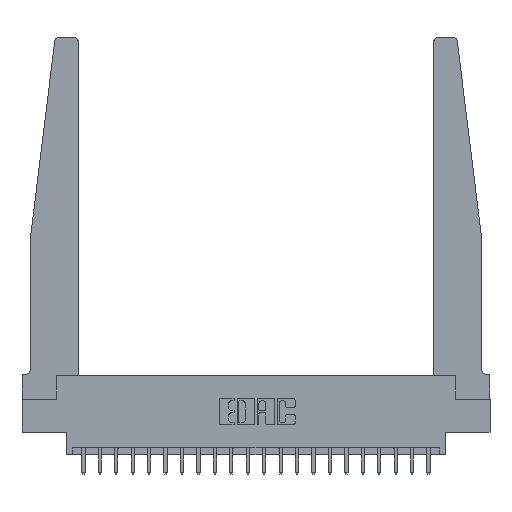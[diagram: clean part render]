
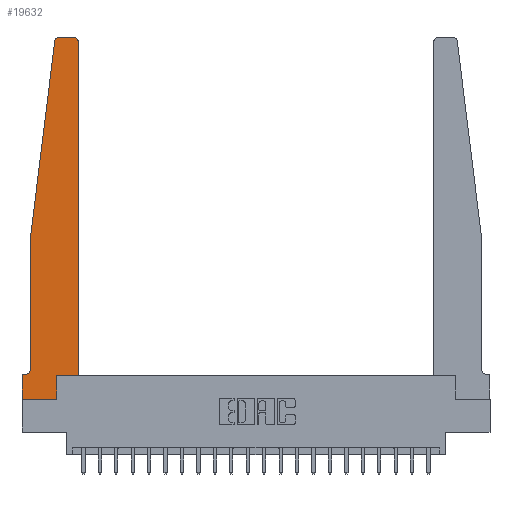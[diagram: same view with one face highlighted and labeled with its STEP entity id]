
A CAD part, top view. The second image highlights one B-rep face of the part: STEP entity #19632.
In plain terms, the highlighted planar face has unit normal (0, 0, 1).
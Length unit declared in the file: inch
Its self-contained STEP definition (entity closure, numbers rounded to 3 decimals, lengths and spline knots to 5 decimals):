
#155 = EDGE_CURVE ( 'NONE', #15139, #5308, #11760, .T. ) ;
#299 = ORIENTED_EDGE ( 'NONE', *, *, #3177, .T. ) ;
#347 = ORIENTED_EDGE ( 'NONE', *, *, #19685, .T. ) ;
#627 = VERTEX_POINT ( 'NONE', #21850 ) ;
#739 = ORIENTED_EDGE ( 'NONE', *, *, #18659, .T. ) ;
#1075 = DIRECTION ( 'NONE',  ( -1., 0., 0. ) ) ;
#1211 = CARTESIAN_POINT ( 'NONE',  ( 0.25, 2.75, 0.37 ) ) ;
#1256 = DIRECTION ( 'NONE',  ( 1., 0., 0. ) ) ;
#1295 = VECTOR ( 'NONE', #15634, 39.37008 ) ;
#1344 = DIRECTION ( 'NONE',  ( -0.122, -0.992, 0. ) ) ;
#1423 = VECTOR ( 'NONE', #5799, 39.37008 ) ;
#1841 = EDGE_CURVE ( 'NONE', #19586, #11223, #8294, .T. ) ;
#2174 = CARTESIAN_POINT ( 'NONE',  ( 0.27653, 2.75, 0.37 ) ) ;
#2571 = VECTOR ( 'NONE', #12663, 39.37008 ) ;
#2574 = LINE ( 'NONE', #14604, #6746 ) ;
#2697 = CARTESIAN_POINT ( 'NONE',  ( 0., 0., 0.37 ) ) ;
#2795 = ORIENTED_EDGE ( 'NONE', *, *, #12098, .T. ) ;
#2828 = EDGE_CURVE ( 'NONE', #16795, #3503, #19050, .T. ) ;
#3177 = EDGE_CURVE ( 'NONE', #13817, #21384, #4140, .T. ) ;
#3387 = ORIENTED_EDGE ( 'NONE', *, *, #6261, .T. ) ;
#3472 = CARTESIAN_POINT ( 'NONE',  ( 0.24675, 2.72367, 0.37 ) ) ;
#3503 = VERTEX_POINT ( 'NONE', #15905 ) ;
#3521 = ORIENTED_EDGE ( 'NONE', *, *, #12812, .T. ) ;
#3889 = DIRECTION ( 'NONE',  ( 1., 0., 0. ) ) ;
#4140 = LINE ( 'NONE', #8401, #17217 ) ;
#4718 = EDGE_LOOP ( 'NONE', ( #5007, #3387, #2795, #13019, #3521, #19135, #5939, #299, #347, #12389, #6267, #739 ) ) ;
#4885 = CARTESIAN_POINT ( 'NONE',  ( 0.065, 0.1875, 0.37 ) ) ;
#5007 = ORIENTED_EDGE ( 'NONE', *, *, #155, .T. ) ;
#5148 = VERTEX_POINT ( 'NONE', #3472 ) ;
#5308 = VERTEX_POINT ( 'NONE', #2174 ) ;
#5482 = CARTESIAN_POINT ( 'NONE',  ( 0., 0., 0.37 ) ) ;
#5781 = LINE ( 'NONE', #16782, #18746 ) ;
#5799 = DIRECTION ( 'NONE',  ( 0., -1., 0. ) ) ;
#5852 = CARTESIAN_POINT ( 'NONE',  ( 0.065, 1.25, 0.37 ) ) ;
#5927 = EDGE_CURVE ( 'NONE', #627, #13817, #10507, .T. ) ;
#5939 = ORIENTED_EDGE ( 'NONE', *, *, #5927, .T. ) ;
#5998 = CARTESIAN_POINT ( 'NONE',  ( 0.425, 0.18, 0.37 ) ) ;
#6261 = EDGE_CURVE ( 'NONE', #5308, #5148, #9170, .T. ) ;
#6266 = CIRCLE ( 'NONE', #16743, 0.03 ) ;
#6267 = ORIENTED_EDGE ( 'NONE', *, *, #8248, .T. ) ;
#6746 = VECTOR ( 'NONE', #16293, 39.37008 ) ;
#7535 = CARTESIAN_POINT ( 'NONE',  ( 0.425, 2.72, 0.37 ) ) ;
#7791 = AXIS2_PLACEMENT_3D ( 'NONE', #8020, #19778, #9748 ) ;
#8020 = CARTESIAN_POINT ( 'NONE',  ( 0.27653, 2.72, 0.37 ) ) ;
#8248 = EDGE_CURVE ( 'NONE', #11223, #10106, #2574, .T. ) ;
#8294 = LINE ( 'NONE', #11623, #8834 ) ;
#8401 = CARTESIAN_POINT ( 'NONE',  ( 0., 0., 0.37 ) ) ;
#8424 = DIRECTION ( 'NONE',  ( -1., 0., 0. ) ) ;
#8834 = VECTOR ( 'NONE', #13326, 39.37008 ) ;
#9151 = FACE_OUTER_BOUND ( 'NONE', #4718, .T. ) ;
#9170 = CIRCLE ( 'NONE', #7791, 0.03 ) ;
#9748 = DIRECTION ( 'NONE',  ( 1., 0., 0. ) ) ;
#10022 = AXIS2_PLACEMENT_3D ( 'NONE', #21387, #11417, #1075 ) ;
#10039 = CIRCLE ( 'NONE', #10022, 0.05 ) ;
#10106 = VERTEX_POINT ( 'NONE', #7535 ) ;
#10124 = DIRECTION ( 'NONE',  ( 1., 0., 0. ) ) ;
#10507 = LINE ( 'NONE', #5482, #1295 ) ;
#10741 = PLANE ( 'NONE',  #15466 ) ;
#10961 = DIRECTION ( 'NONE',  ( 0., 1., 0. ) ) ;
#11223 = VERTEX_POINT ( 'NONE', #5998 ) ;
#11417 = DIRECTION ( 'NONE',  ( 0., 0., -1. ) ) ;
#11590 = DIRECTION ( 'NONE',  ( 0., 0., 1. ) ) ;
#11623 = CARTESIAN_POINT ( 'NONE',  ( 0.425, 0.18, 0.37 ) ) ;
#11760 = LINE ( 'NONE', #1211, #2571 ) ;
#12098 = EDGE_CURVE ( 'NONE', #5148, #16795, #5781, .T. ) ;
#12130 = EDGE_CURVE ( 'NONE', #17674, #627, #18234, .T. ) ;
#12389 = ORIENTED_EDGE ( 'NONE', *, *, #1841, .T. ) ;
#12440 = CARTESIAN_POINT ( 'NONE',  ( 0., 0.1875, 0.37 ) ) ;
#12663 = DIRECTION ( 'NONE',  ( -1., 0., 0. ) ) ;
#12812 = EDGE_CURVE ( 'NONE', #3503, #17674, #10039, .T. ) ;
#13019 = ORIENTED_EDGE ( 'NONE', *, *, #2828, .T. ) ;
#13326 = DIRECTION ( 'NONE',  ( 1., 0., 0. ) ) ;
#13752 = VECTOR ( 'NONE', #8424, 39.37008 ) ;
#13817 = VERTEX_POINT ( 'NONE', #2697 ) ;
#14074 = CARTESIAN_POINT ( 'NONE',  ( 0.2605, 0.18, 0.37 ) ) ;
#14142 = DIRECTION ( 'NONE',  ( 0., 0., 1. ) ) ;
#14604 = CARTESIAN_POINT ( 'NONE',  ( 0.425, 0.18, 0.37 ) ) ;
#15139 = VERTEX_POINT ( 'NONE', #19912 ) ;
#15466 = AXIS2_PLACEMENT_3D ( 'NONE', #12440, #14142, #3889 ) ;
#15634 = DIRECTION ( 'NONE',  ( 0., -1., 0. ) ) ;
#15905 = CARTESIAN_POINT ( 'NONE',  ( 0.065, 0.2375, 0.37 ) ) ;
#16293 = DIRECTION ( 'NONE',  ( 0., 1., 0. ) ) ;
#16538 = VECTOR ( 'NONE', #10961, 39.37008 ) ;
#16743 = AXIS2_PLACEMENT_3D ( 'NONE', #21565, #11590, #1256 ) ;
#16782 = CARTESIAN_POINT ( 'NONE',  ( 0.065, 1.25, 0.37 ) ) ;
#16795 = VERTEX_POINT ( 'NONE', #5852 ) ;
#17217 = VECTOR ( 'NONE', #10124, 39.37008 ) ;
#17616 = CARTESIAN_POINT ( 'NONE',  ( 0.2605, 0.18, 0.37 ) ) ;
#17674 = VERTEX_POINT ( 'NONE', #21357 ) ;
#18234 = LINE ( 'NONE', #4885, #13752 ) ;
#18659 = EDGE_CURVE ( 'NONE', #10106, #15139, #6266, .T. ) ;
#18746 = VECTOR ( 'NONE', #1344, 39.37008 ) ;
#19050 = LINE ( 'NONE', #19296, #1423 ) ;
#19135 = ORIENTED_EDGE ( 'NONE', *, *, #12130, .T. ) ;
#19296 = CARTESIAN_POINT ( 'NONE',  ( 0.065, 1.25, 0.37 ) ) ;
#19586 = VERTEX_POINT ( 'NONE', #14074 ) ;
#19632 = ADVANCED_FACE ( 'NONE', ( #9151 ), #10741, .T. ) ;
#19685 = EDGE_CURVE ( 'NONE', #21384, #19586, #21407, .T. ) ;
#19778 = DIRECTION ( 'NONE',  ( 0., 0., 1. ) ) ;
#19912 = CARTESIAN_POINT ( 'NONE',  ( 0.395, 2.75, 0.37 ) ) ;
#20157 = CARTESIAN_POINT ( 'NONE',  ( 0.2605, 0., 0.37 ) ) ;
#21357 = CARTESIAN_POINT ( 'NONE',  ( 0.015, 0.1875, 0.37 ) ) ;
#21384 = VERTEX_POINT ( 'NONE', #20157 ) ;
#21387 = CARTESIAN_POINT ( 'NONE',  ( 0.015, 0.2375, 0.37 ) ) ;
#21407 = LINE ( 'NONE', #17616, #16538 ) ;
#21565 = CARTESIAN_POINT ( 'NONE',  ( 0.395, 2.72, 0.37 ) ) ;
#21850 = CARTESIAN_POINT ( 'NONE',  ( 0., 0.1875, 0.37 ) ) ;
